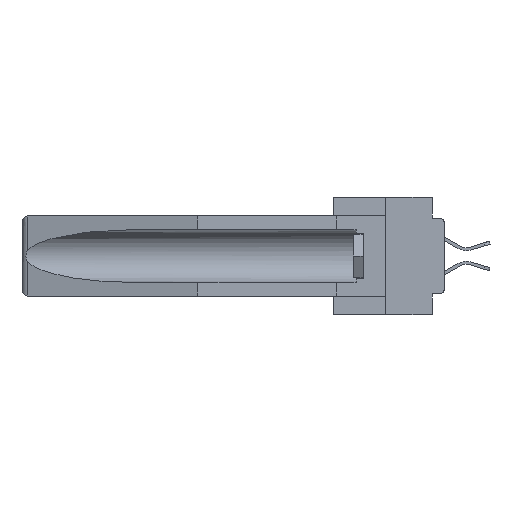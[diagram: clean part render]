
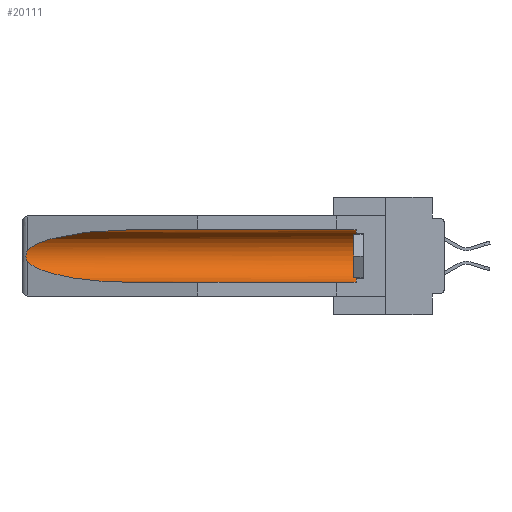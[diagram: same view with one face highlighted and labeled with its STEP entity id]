
A CAD part, left-side view. The second image highlights one B-rep face of the part: STEP entity #20111.
In plain terms, the highlighted cylindrical face has radius 2.857 mm (diameter 5.715 mm), a partial arc.
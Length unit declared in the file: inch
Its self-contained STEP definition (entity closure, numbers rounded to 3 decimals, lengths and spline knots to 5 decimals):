
#414 = VECTOR ( 'NONE', #24834, 39.37008 ) ;
#430 = CARTESIAN_POINT ( 'NONE',  ( 0.21114, 1.30732, -0.284 ) ) ;
#1764 = AXIS2_PLACEMENT_3D ( 'NONE', #13725, #32138, #21575 ) ;
#1896 = LINE ( 'NONE', #22795, #29238 ) ;
#1970 = CARTESIAN_POINT ( 'NONE',  ( 0.155, 1.07973, -0.059 ) ) ;
#2232 = CARTESIAN_POINT ( 'NONE',  ( 0.155, 1.07973, -0.284 ) ) ;
#2975 = CARTESIAN_POINT ( 'NONE',  ( 0.2675, 1.53308, -0.16763 ) ) ;
#4632 = ORIENTED_EDGE ( 'NONE', *, *, #6163, .T. ) ;
#5623 = AXIS2_PLACEMENT_3D ( 'NONE', #28341, #7476, #10560 ) ;
#5882 = CARTESIAN_POINT ( 'NONE',  ( 0.26654, 1.53092, -0.15636 ) ) ;
#6163 = EDGE_CURVE ( 'NONE', #31476, #7818, #32360, .T. ) ;
#6342 = EDGE_LOOP ( 'NONE', ( #15982, #32333, #16425, #31287, #4632, #23818 ) ) ;
#7420 = CARTESIAN_POINT ( 'NONE',  ( 0.26537, 1.52718, -0.14972 ) ) ;
#7476 = DIRECTION ( 'NONE',  ( 0., 1., 0. ) ) ;
#7818 = VERTEX_POINT ( 'NONE', #15724 ) ;
#7923 = EDGE_CURVE ( 'NONE', #20925, #25224, #9673, .T. ) ;
#9673 =( BOUNDED_CURVE ( )  B_SPLINE_CURVE ( 3, ( #21686, #23886, #430, #22176 ),
 .UNSPECIFIED., .F., .F. ) 
 B_SPLINE_CURVE_WITH_KNOTS ( ( 4, 4 ),
 ( 0.1948, 1.5708 ),
 .UNSPECIFIED. ) 
 CURVE ( )  GEOMETRIC_REPRESENTATION_ITEM ( )  RATIONAL_B_SPLINE_CURVE ( ( 1., 0.848, 0.848, 1. ) ) 
 REPRESENTATION_ITEM ( '' )  );
#10560 = DIRECTION ( 'NONE',  ( 0., 0., 1. ) ) ;
#10575 =( BOUNDED_CURVE ( )  B_SPLINE_CURVE ( 3, ( #20607, #20442, #30493, #7420 ),
 .UNSPECIFIED., .F., .F. ) 
 B_SPLINE_CURVE_WITH_KNOTS ( ( 4, 4 ),
 ( 4.71239, 6.08839 ),
 .UNSPECIFIED. ) 
 CURVE ( )  GEOMETRIC_REPRESENTATION_ITEM ( )  RATIONAL_B_SPLINE_CURVE ( ( 1., 0.848, 0.848, 1. ) ) 
 REPRESENTATION_ITEM ( '' )  );
#13085 = EDGE_CURVE ( 'NONE', #7818, #25540, #29956, .T. ) ;
#13288 = CARTESIAN_POINT ( 'NONE',  ( 0.26597, 1.5296, -0.19026 ) ) ;
#13459 = CARTESIAN_POINT ( 'NONE',  ( 0.2675, 1.53308, -0.17534 ) ) ;
#13725 = CARTESIAN_POINT ( 'NONE',  ( 0.155, 0.126, -0.1715 ) ) ;
#14433 = DIRECTION ( 'NONE',  ( 0., 1., 0. ) ) ;
#15724 = CARTESIAN_POINT ( 'NONE',  ( 0.155, 0.126, -0.059 ) ) ;
#15982 = ORIENTED_EDGE ( 'NONE', *, *, #28402, .T. ) ;
#16351 = CARTESIAN_POINT ( 'NONE',  ( 0.26537, 1.52718, -0.19328 ) ) ;
#16425 = ORIENTED_EDGE ( 'NONE', *, *, #7923, .T. ) ;
#16985 = CARTESIAN_POINT ( 'NONE',  ( 0.155, -0.30754, -0.059 ) ) ;
#18461 = VERTEX_POINT ( 'NONE', #27409 ) ;
#18750 = CARTESIAN_POINT ( 'NONE',  ( 0.26655, 1.53094, -0.18657 ) ) ;
#19460 = CARTESIAN_POINT ( 'NONE',  ( 0.155, 0.126, -0.284 ) ) ;
#20111 = ADVANCED_FACE ( 'NONE', ( #33776 ), #23694, .F. ) ;
#20442 = CARTESIAN_POINT ( 'NONE',  ( 0.21114, 1.30732, -0.059 ) ) ;
#20607 = CARTESIAN_POINT ( 'NONE',  ( 0.155, 1.07973, -0.059 ) ) ;
#20925 = VERTEX_POINT ( 'NONE', #30814 ) ;
#21575 = DIRECTION ( 'NONE',  ( 0., 0., 1. ) ) ;
#21652 = CARTESIAN_POINT ( 'NONE',  ( 0.26537, 1.52718, -0.14972 ) ) ;
#21686 = CARTESIAN_POINT ( 'NONE',  ( 0.26537, 1.52718, -0.19328 ) ) ;
#22176 = CARTESIAN_POINT ( 'NONE',  ( 0.155, 1.07973, -0.284 ) ) ;
#22186 = EDGE_CURVE ( 'NONE', #31476, #25224, #1896, .T. ) ;
#22795 = CARTESIAN_POINT ( 'NONE',  ( 0.155, -0.30754, -0.284 ) ) ;
#23694 = CYLINDRICAL_SURFACE ( 'NONE', #5623, 0.1125 ) ;
#23818 = ORIENTED_EDGE ( 'NONE', *, *, #13085, .T. ) ;
#23886 = CARTESIAN_POINT ( 'NONE',  ( 0.25451, 1.48313, -0.24835 ) ) ;
#24468 = EDGE_CURVE ( 'NONE', #18461, #20925, #32731, .T. ) ;
#24834 = DIRECTION ( 'NONE',  ( 0., 1., 0. ) ) ;
#25224 = VERTEX_POINT ( 'NONE', #2232 ) ;
#25540 = VERTEX_POINT ( 'NONE', #1970 ) ;
#26426 = CARTESIAN_POINT ( 'NONE',  ( 0.2673, 1.5327, -0.16383 ) ) ;
#26596 = CARTESIAN_POINT ( 'NONE',  ( 0.26597, 1.52961, -0.15275 ) ) ;
#27409 = CARTESIAN_POINT ( 'NONE',  ( 0.26537, 1.52718, -0.14972 ) ) ;
#28341 = CARTESIAN_POINT ( 'NONE',  ( 0.155, -0.30754, -0.1715 ) ) ;
#28402 = EDGE_CURVE ( 'NONE', #25540, #18461, #10575, .T. ) ;
#29238 = VECTOR ( 'NONE', #14433, 39.37008 ) ;
#29956 = LINE ( 'NONE', #16985, #414 ) ;
#30493 = CARTESIAN_POINT ( 'NONE',  ( 0.25451, 1.48313, -0.09465 ) ) ;
#30814 = CARTESIAN_POINT ( 'NONE',  ( 0.26537, 1.52718, -0.19328 ) ) ;
#31287 = ORIENTED_EDGE ( 'NONE', *, *, #22186, .F. ) ;
#31476 = VERTEX_POINT ( 'NONE', #19460 ) ;
#31877 = CARTESIAN_POINT ( 'NONE',  ( 0.2673, 1.53269, -0.17917 ) ) ;
#32138 = DIRECTION ( 'NONE',  ( 0., -1., 0. ) ) ;
#32333 = ORIENTED_EDGE ( 'NONE', *, *, #24468, .T. ) ;
#32360 = CIRCLE ( 'NONE', #1764, 0.1125 ) ;
#32731 = B_SPLINE_CURVE_WITH_KNOTS ( 'NONE', 3,
 ( #21652, #26596, #5882, #26426, #2975, #13459, #31877, #18750, #13288, #16351 ),
 .UNSPECIFIED., .F., .F.,
 ( 4, 2, 2, 2, 4 ),
 ( 0., 0.00029, 0.00058, 0.00087, 0.00117 ),
 .UNSPECIFIED. ) ;
#33776 = FACE_OUTER_BOUND ( 'NONE', #6342, .T. ) ;
